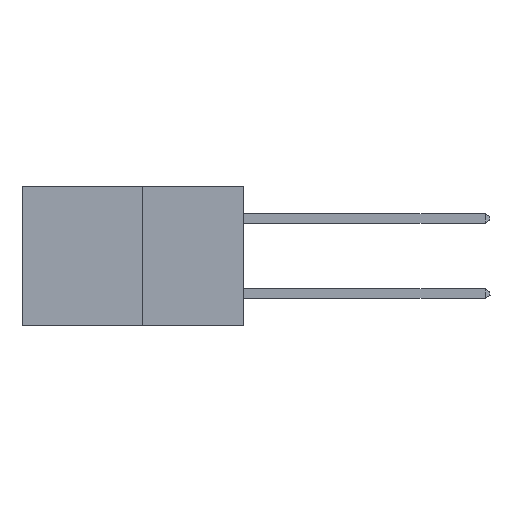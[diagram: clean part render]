
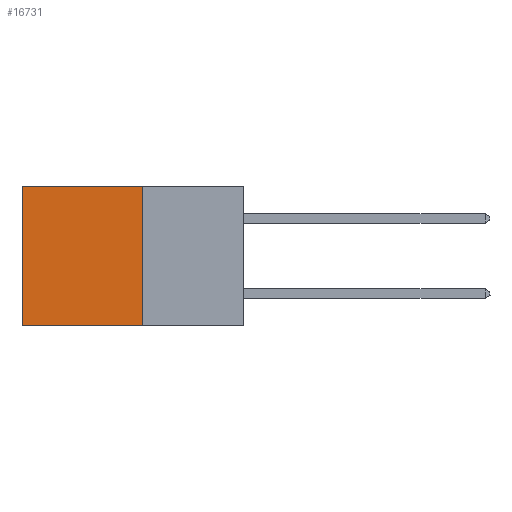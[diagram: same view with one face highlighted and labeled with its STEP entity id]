
A CAD part, left-side view. The second image highlights one B-rep face of the part: STEP entity #16731.
In plain terms, the highlighted planar face has unit normal (-1, 0, 0).
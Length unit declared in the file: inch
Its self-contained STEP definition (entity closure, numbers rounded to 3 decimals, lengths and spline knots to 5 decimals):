
#639 = CARTESIAN_POINT ( 'NONE',  ( 0.277, 0.27, 0. ) ) ;
#2288 = CARTESIAN_POINT ( 'NONE',  ( 0.277, 0.27, 0. ) ) ;
#2672 = ORIENTED_EDGE ( 'NONE', *, *, #15796, .T. ) ;
#3483 = VECTOR ( 'NONE', #14290, 39.37008 ) ;
#3530 = FACE_OUTER_BOUND ( 'NONE', #23233, .T. ) ;
#3677 = DIRECTION ( 'NONE',  ( 1., 0., 0. ) ) ;
#5087 = EDGE_CURVE ( 'NONE', #15680, #22566, #17315, .T. ) ;
#6533 = DIRECTION ( 'NONE',  ( 0., 1., 0. ) ) ;
#7269 = CARTESIAN_POINT ( 'NONE',  ( 0.277, 0.59, -0.37 ) ) ;
#7335 = LINE ( 'NONE', #7269, #23348 ) ;
#7987 = CARTESIAN_POINT ( 'NONE',  ( 0.277, 0.59, 0. ) ) ;
#9391 = VECTOR ( 'NONE', #6533, 39.37008 ) ;
#9569 = ORIENTED_EDGE ( 'NONE', *, *, #14328, .T. ) ;
#10994 = AXIS2_PLACEMENT_3D ( 'NONE', #24766, #3677, #17277 ) ;
#12098 = EDGE_CURVE ( 'NONE', #22566, #14857, #13217, .T. ) ;
#12625 = CARTESIAN_POINT ( 'NONE',  ( 0.277, 0.27, -0.37 ) ) ;
#13217 = LINE ( 'NONE', #23876, #3483 ) ;
#13241 = VERTEX_POINT ( 'NONE', #7987 ) ;
#14290 = DIRECTION ( 'NONE',  ( 0., 1., 0. ) ) ;
#14328 = EDGE_CURVE ( 'NONE', #13241, #14857, #7335, .T. ) ;
#14857 = VERTEX_POINT ( 'NONE', #16400 ) ;
#15069 = DIRECTION ( 'NONE',  ( 0., 0., -1. ) ) ;
#15337 = ORIENTED_EDGE ( 'NONE', *, *, #12098, .F. ) ;
#15680 = VERTEX_POINT ( 'NONE', #2288 ) ;
#15796 = EDGE_CURVE ( 'NONE', #15680, #13241, #24719, .T. ) ;
#16400 = CARTESIAN_POINT ( 'NONE',  ( 0.277, 0.59, -0.37 ) ) ;
#16731 = ADVANCED_FACE ( 'NONE', ( #3530 ), #24850, .F. ) ;
#16865 = CARTESIAN_POINT ( 'NONE',  ( 0.277, 0.27, -0.37 ) ) ;
#17277 = DIRECTION ( 'NONE',  ( 0., 0., -1. ) ) ;
#17315 = LINE ( 'NONE', #16865, #17954 ) ;
#17954 = VECTOR ( 'NONE', #15069, 39.37008 ) ;
#21502 = ORIENTED_EDGE ( 'NONE', *, *, #5087, .F. ) ;
#22566 = VERTEX_POINT ( 'NONE', #12625 ) ;
#23233 = EDGE_LOOP ( 'NONE', ( #9569, #15337, #21502, #2672 ) ) ;
#23348 = VECTOR ( 'NONE', #24601, 39.37008 ) ;
#23876 = CARTESIAN_POINT ( 'NONE',  ( 0.277, 0.27, -0.37 ) ) ;
#24601 = DIRECTION ( 'NONE',  ( 0., 0., -1. ) ) ;
#24719 = LINE ( 'NONE', #639, #9391 ) ;
#24766 = CARTESIAN_POINT ( 'NONE',  ( 0.277, 0.27, -0.37 ) ) ;
#24850 = PLANE ( 'NONE',  #10994 ) ;
